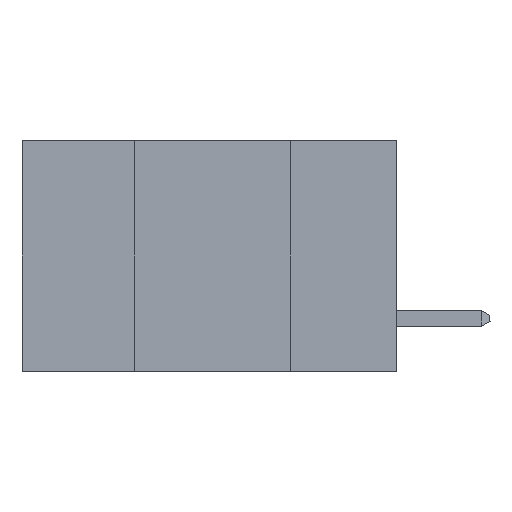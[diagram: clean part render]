
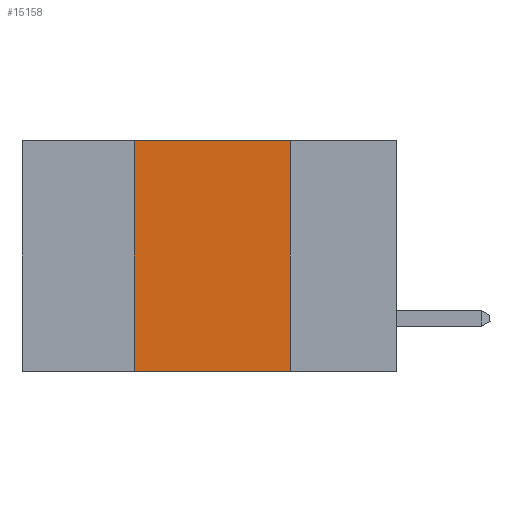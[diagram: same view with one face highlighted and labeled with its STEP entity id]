
A CAD part, left-side view. The second image highlights one B-rep face of the part: STEP entity #15158.
In plain terms, the highlighted planar face has unit normal (-1, 0, 0).
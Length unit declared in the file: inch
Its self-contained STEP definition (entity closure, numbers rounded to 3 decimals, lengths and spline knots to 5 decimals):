
#889 = LINE ( 'NONE', #4607, #14382 ) ;
#1401 = DIRECTION ( 'NONE',  ( 1., 0., 0. ) ) ;
#1538 = CARTESIAN_POINT ( 'NONE',  ( 0., 0.17, 0. ) ) ;
#2524 = EDGE_CURVE ( 'NONE', #10507, #3050, #15190, .T. ) ;
#2695 = CARTESIAN_POINT ( 'NONE',  ( 0., 0.6, 0. ) ) ;
#3050 = VERTEX_POINT ( 'NONE', #9116 ) ;
#4607 = CARTESIAN_POINT ( 'NONE',  ( 0., 0.17, 0. ) ) ;
#4996 = EDGE_CURVE ( 'NONE', #10507, #8497, #19570, .T. ) ;
#5903 = ORIENTED_EDGE ( 'NONE', *, *, #2524, .T. ) ;
#6084 = ORIENTED_EDGE ( 'NONE', *, *, #19110, .F. ) ;
#6600 = CARTESIAN_POINT ( 'NONE',  ( 0., 0.6, -0.37 ) ) ;
#6897 = VECTOR ( 'NONE', #9368, 39.37008 ) ;
#7947 = CARTESIAN_POINT ( 'NONE',  ( 0., 0.42, 0. ) ) ;
#8497 = VERTEX_POINT ( 'NONE', #10153 ) ;
#8777 = CARTESIAN_POINT ( 'NONE',  ( 0., 0.42, -0.37 ) ) ;
#9116 = CARTESIAN_POINT ( 'NONE',  ( 0., 0.17, -0.37 ) ) ;
#9160 = FACE_OUTER_BOUND ( 'NONE', #16472, .T. ) ;
#9368 = DIRECTION ( 'NONE',  ( 0., -1., 0. ) ) ;
#9522 = VERTEX_POINT ( 'NONE', #1538 ) ;
#10153 = CARTESIAN_POINT ( 'NONE',  ( 0., 0.42, 0. ) ) ;
#10507 = VERTEX_POINT ( 'NONE', #8777 ) ;
#10790 = ORIENTED_EDGE ( 'NONE', *, *, #4996, .F. ) ;
#12423 = DIRECTION ( 'NONE',  ( 0., 0., -1. ) ) ;
#13991 = DIRECTION ( 'NONE',  ( 0., 0., -1. ) ) ;
#14382 = VECTOR ( 'NONE', #13991, 39.37008 ) ;
#15158 = ADVANCED_FACE ( 'NONE', ( #9160 ), #17040, .F. ) ;
#15190 = LINE ( 'NONE', #6600, #6897 ) ;
#15231 = DIRECTION ( 'NONE',  ( 0., -1., 0. ) ) ;
#16063 = LINE ( 'NONE', #2695, #20175 ) ;
#16378 = AXIS2_PLACEMENT_3D ( 'NONE', #18607, #1401, #12423 ) ;
#16456 = ORIENTED_EDGE ( 'NONE', *, *, #17893, .F. ) ;
#16472 = EDGE_LOOP ( 'NONE', ( #16456, #6084, #10790, #5903 ) ) ;
#17040 = PLANE ( 'NONE',  #16378 ) ;
#17893 = EDGE_CURVE ( 'NONE', #9522, #3050, #889, .T. ) ;
#18607 = CARTESIAN_POINT ( 'NONE',  ( 0., 0.6, 0. ) ) ;
#19085 = VECTOR ( 'NONE', #19728, 39.37008 ) ;
#19110 = EDGE_CURVE ( 'NONE', #8497, #9522, #16063, .T. ) ;
#19570 = LINE ( 'NONE', #7947, #19085 ) ;
#19728 = DIRECTION ( 'NONE',  ( 0., 0., 1. ) ) ;
#20175 = VECTOR ( 'NONE', #15231, 39.37008 ) ;
